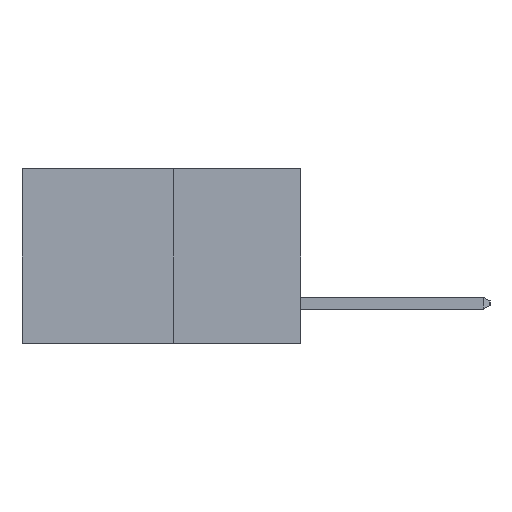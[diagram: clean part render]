
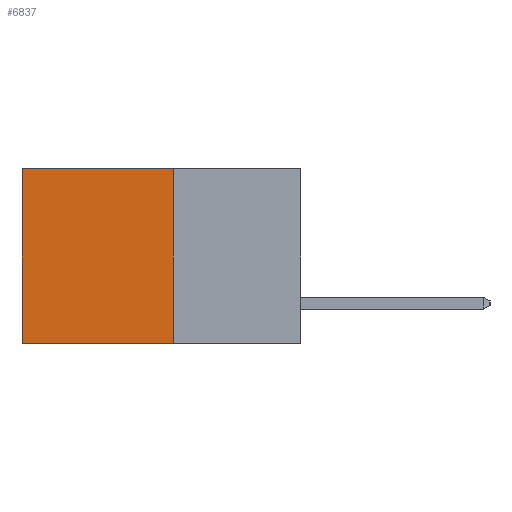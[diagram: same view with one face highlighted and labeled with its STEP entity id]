
A CAD part, left-side view. The second image highlights one B-rep face of the part: STEP entity #6837.
In plain terms, the highlighted planar face has unit normal (-1, 0, 0).
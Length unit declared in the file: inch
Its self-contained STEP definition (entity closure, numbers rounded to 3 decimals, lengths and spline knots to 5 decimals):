
#11 = LINE ( 'NONE', #2760, #7785 ) ;
#190 = VECTOR ( 'NONE', #3697, 39.37008 ) ;
#208 = PLANE ( 'NONE',  #4134 ) ;
#468 = VECTOR ( 'NONE', #8292, 39.37008 ) ;
#643 = CARTESIAN_POINT ( 'NONE',  ( 0.277, 0.27, -0.37 ) ) ;
#1681 = DIRECTION ( 'NONE',  ( 0., 0., -1. ) ) ;
#2084 = DIRECTION ( 'NONE',  ( 0., 1., 0. ) ) ;
#2391 = DIRECTION ( 'NONE',  ( 1., 0., 0. ) ) ;
#2523 = VERTEX_POINT ( 'NONE', #2875 ) ;
#2721 = LINE ( 'NONE', #643, #4422 ) ;
#2760 = CARTESIAN_POINT ( 'NONE',  ( 0.277, 0.59, -0.37 ) ) ;
#2875 = CARTESIAN_POINT ( 'NONE',  ( 0.277, 0.59, -0.37 ) ) ;
#2930 = VERTEX_POINT ( 'NONE', #6568 ) ;
#3103 = CARTESIAN_POINT ( 'NONE',  ( 0.277, 0.27, -0.37 ) ) ;
#3152 = CARTESIAN_POINT ( 'NONE',  ( 0.277, 0.27, 0. ) ) ;
#3184 = CARTESIAN_POINT ( 'NONE',  ( 0.277, 0.27, -0.37 ) ) ;
#3354 = VERTEX_POINT ( 'NONE', #4096 ) ;
#3554 = CARTESIAN_POINT ( 'NONE',  ( 0.277, 0.27, -0.37 ) ) ;
#3623 = EDGE_CURVE ( 'NONE', #2930, #3354, #6047, .T. ) ;
#3697 = DIRECTION ( 'NONE',  ( 0., 1., 0. ) ) ;
#4096 = CARTESIAN_POINT ( 'NONE',  ( 0.277, 0.59, 0. ) ) ;
#4134 = AXIS2_PLACEMENT_3D ( 'NONE', #3103, #2391, #1681 ) ;
#4422 = VECTOR ( 'NONE', #2084, 39.37008 ) ;
#4470 = ORIENTED_EDGE ( 'NONE', *, *, #7526, .F. ) ;
#6038 = ORIENTED_EDGE ( 'NONE', *, *, #3623, .T. ) ;
#6047 = LINE ( 'NONE', #3152, #190 ) ;
#6443 = FACE_OUTER_BOUND ( 'NONE', #7641, .T. ) ;
#6507 = ORIENTED_EDGE ( 'NONE', *, *, #8516, .F. ) ;
#6568 = CARTESIAN_POINT ( 'NONE',  ( 0.277, 0.27, 0. ) ) ;
#6837 = ADVANCED_FACE ( 'NONE', ( #6443 ), #208, .F. ) ;
#7150 = EDGE_CURVE ( 'NONE', #3354, #2523, #11, .T. ) ;
#7526 = EDGE_CURVE ( 'NONE', #2930, #7887, #7779, .T. ) ;
#7641 = EDGE_LOOP ( 'NONE', ( #7842, #6507, #4470, #6038 ) ) ;
#7779 = LINE ( 'NONE', #3184, #468 ) ;
#7785 = VECTOR ( 'NONE', #7874, 39.37008 ) ;
#7842 = ORIENTED_EDGE ( 'NONE', *, *, #7150, .T. ) ;
#7874 = DIRECTION ( 'NONE',  ( 0., 0., -1. ) ) ;
#7887 = VERTEX_POINT ( 'NONE', #3554 ) ;
#8292 = DIRECTION ( 'NONE',  ( 0., 0., -1. ) ) ;
#8516 = EDGE_CURVE ( 'NONE', #7887, #2523, #2721, .T. ) ;
